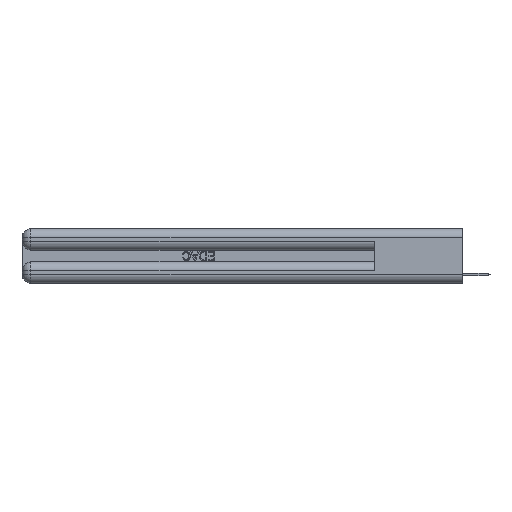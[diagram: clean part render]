
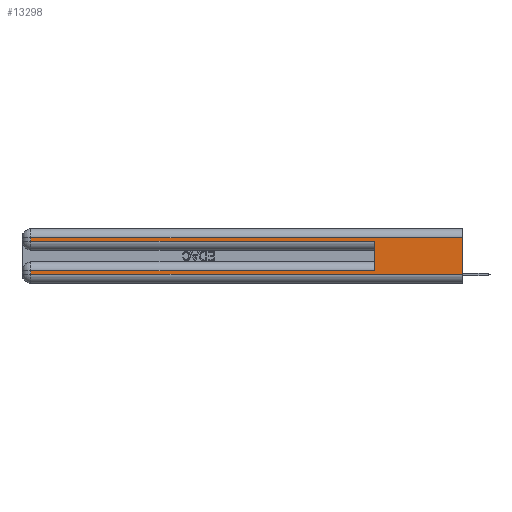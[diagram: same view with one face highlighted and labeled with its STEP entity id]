
A CAD part, left-side view. The second image highlights one B-rep face of the part: STEP entity #13298.
In plain terms, the highlighted planar face has unit normal (-1, 0, 0).
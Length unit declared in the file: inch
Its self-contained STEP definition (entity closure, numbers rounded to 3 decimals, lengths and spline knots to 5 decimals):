
#1057 = ORIENTED_EDGE ( 'NONE', *, *, #10037, .T. ) ;
#1188 = VECTOR ( 'NONE', #13479, 39.37008 ) ;
#1341 = VECTOR ( 'NONE', #23388, 39.37008 ) ;
#2105 = LINE ( 'NONE', #10466, #13526 ) ;
#2340 = LINE ( 'NONE', #5249, #9268 ) ;
#2508 = VECTOR ( 'NONE', #20312, 39.37008 ) ;
#2957 = CARTESIAN_POINT ( 'NONE',  ( 0., 0.6, 0.145 ) ) ;
#3002 = VECTOR ( 'NONE', #16196, 39.37008 ) ;
#4437 = EDGE_CURVE ( 'NONE', #27255, #31546, #20428, .T. ) ;
#5191 = CARTESIAN_POINT ( 'NONE',  ( 0., 0., 0.085 ) ) ;
#5249 = CARTESIAN_POINT ( 'NONE',  ( 0., 0., 0.06 ) ) ;
#6808 = AXIS2_PLACEMENT_3D ( 'NONE', #13601, #18515, #23681 ) ;
#7493 = CARTESIAN_POINT ( 'NONE',  ( 0., 2.94, 0.37 ) ) ;
#7942 = CARTESIAN_POINT ( 'NONE',  ( 0., 0.6, 0.285 ) ) ;
#7958 = DIRECTION ( 'NONE',  ( 0., 0., -1. ) ) ;
#8091 = VERTEX_POINT ( 'NONE', #8983 ) ;
#8261 = EDGE_CURVE ( 'NONE', #26161, #27255, #16043, .T. ) ;
#8274 = EDGE_CURVE ( 'NONE', #32145, #8977, #13176, .T. ) ;
#8977 = VERTEX_POINT ( 'NONE', #7942 ) ;
#8983 = CARTESIAN_POINT ( 'NONE',  ( 0., 2.94, 0.31 ) ) ;
#9255 = EDGE_CURVE ( 'NONE', #15260, #33328, #10276, .T. ) ;
#9268 = VECTOR ( 'NONE', #21167, 39.37008 ) ;
#10037 = EDGE_CURVE ( 'NONE', #8091, #32145, #2105, .T. ) ;
#10276 = LINE ( 'NONE', #12793, #2508 ) ;
#10466 = CARTESIAN_POINT ( 'NONE',  ( 0., 2.94, 0.37 ) ) ;
#11717 = EDGE_CURVE ( 'NONE', #15260, #8091, #33018, .T. ) ;
#12357 = VECTOR ( 'NONE', #20523, 39.37008 ) ;
#12793 = CARTESIAN_POINT ( 'NONE',  ( 0., 0., 0.37 ) ) ;
#13176 = LINE ( 'NONE', #25665, #12357 ) ;
#13298 = ADVANCED_FACE ( 'NONE', ( #24787 ), #28556, .F. ) ;
#13479 = DIRECTION ( 'NONE',  ( 0., 1., 0. ) ) ;
#13526 = VECTOR ( 'NONE', #7958, 39.37008 ) ;
#13601 = CARTESIAN_POINT ( 'NONE',  ( 0., 0., 0.37 ) ) ;
#15061 = ORIENTED_EDGE ( 'NONE', *, *, #8261, .T. ) ;
#15260 = VERTEX_POINT ( 'NONE', #25637 ) ;
#16043 = LINE ( 'NONE', #5191, #1341 ) ;
#16196 = DIRECTION ( 'NONE',  ( 0., 0., 1. ) ) ;
#16920 = CARTESIAN_POINT ( 'NONE',  ( 0., 2.94, 0.085 ) ) ;
#17856 = CARTESIAN_POINT ( 'NONE',  ( 0., 0.6, 0.085 ) ) ;
#18515 = DIRECTION ( 'NONE',  ( 1., 0., 0. ) ) ;
#18558 = ORIENTED_EDGE ( 'NONE', *, *, #4437, .T. ) ;
#19765 = ORIENTED_EDGE ( 'NONE', *, *, #9255, .F. ) ;
#19770 = ORIENTED_EDGE ( 'NONE', *, *, #11717, .T. ) ;
#20312 = DIRECTION ( 'NONE',  ( 0., 0., -1. ) ) ;
#20428 = LINE ( 'NONE', #7493, #31449 ) ;
#20523 = DIRECTION ( 'NONE',  ( 0., -1., 0. ) ) ;
#20646 = DIRECTION ( 'NONE',  ( 0., 0., -1. ) ) ;
#21167 = DIRECTION ( 'NONE',  ( 0., -1., 0. ) ) ;
#21627 = EDGE_CURVE ( 'NONE', #31546, #33328, #2340, .T. ) ;
#22029 = CARTESIAN_POINT ( 'NONE',  ( 0., 2.94, 0.285 ) ) ;
#23388 = DIRECTION ( 'NONE',  ( 0., 1., 0. ) ) ;
#23508 = EDGE_CURVE ( 'NONE', #26161, #8977, #29904, .T. ) ;
#23681 = DIRECTION ( 'NONE',  ( 0., 0., -1. ) ) ;
#24545 = ORIENTED_EDGE ( 'NONE', *, *, #8274, .T. ) ;
#24787 = FACE_OUTER_BOUND ( 'NONE', #25181, .T. ) ;
#25181 = EDGE_LOOP ( 'NONE', ( #19765, #19770, #1057, #24545, #32187, #15061, #18558, #30226 ) ) ;
#25637 = CARTESIAN_POINT ( 'NONE',  ( 0., 0., 0.31 ) ) ;
#25665 = CARTESIAN_POINT ( 'NONE',  ( 0., 0., 0.285 ) ) ;
#26161 = VERTEX_POINT ( 'NONE', #17856 ) ;
#26641 = CARTESIAN_POINT ( 'NONE',  ( 0., 0., 0.31 ) ) ;
#27255 = VERTEX_POINT ( 'NONE', #16920 ) ;
#28556 = PLANE ( 'NONE',  #6808 ) ;
#29293 = CARTESIAN_POINT ( 'NONE',  ( 0., 2.94, 0.06 ) ) ;
#29885 = CARTESIAN_POINT ( 'NONE',  ( 0., 0., 0.06 ) ) ;
#29904 = LINE ( 'NONE', #2957, #3002 ) ;
#30226 = ORIENTED_EDGE ( 'NONE', *, *, #21627, .T. ) ;
#31449 = VECTOR ( 'NONE', #20646, 39.37008 ) ;
#31546 = VERTEX_POINT ( 'NONE', #29293 ) ;
#32145 = VERTEX_POINT ( 'NONE', #22029 ) ;
#32187 = ORIENTED_EDGE ( 'NONE', *, *, #23508, .F. ) ;
#33018 = LINE ( 'NONE', #26641, #1188 ) ;
#33328 = VERTEX_POINT ( 'NONE', #29885 ) ;
